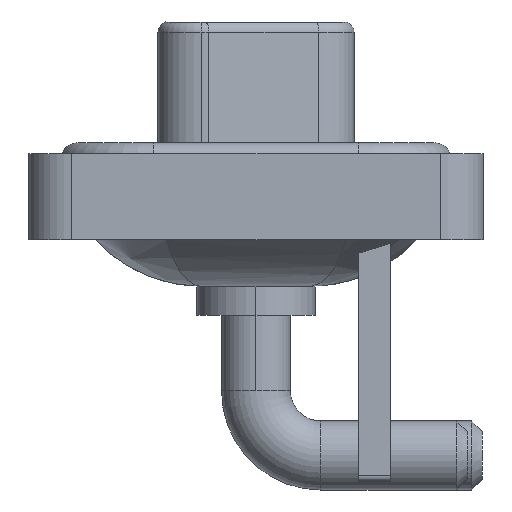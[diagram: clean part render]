
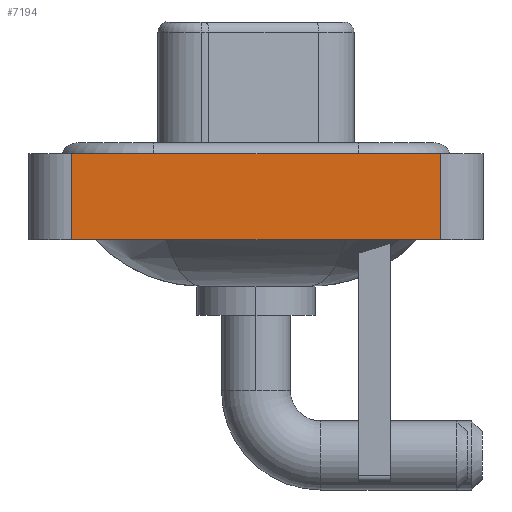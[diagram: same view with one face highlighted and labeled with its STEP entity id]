
A CAD part, left-side view. The second image highlights one B-rep face of the part: STEP entity #7194.
In plain terms, the highlighted planar face has unit normal (-1, 0, 0).
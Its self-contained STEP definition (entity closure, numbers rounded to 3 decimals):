
#233 = CARTESIAN_POINT ( 'NONE',  ( -7.3, -8.55, 0.4 ) ) ;
#431 = CARTESIAN_POINT ( 'NONE',  ( -7.3, 8.55, -3.6 ) ) ;
#856 = DIRECTION ( 'NONE',  ( 0., 0., 1. ) ) ;
#1023 = VECTOR ( 'NONE', #856, 1000. ) ;
#2092 = AXIS2_PLACEMENT_3D ( 'NONE', #8544, #11675, #17555 ) ;
#2222 = CARTESIAN_POINT ( 'NONE',  ( -7.3, -8.55, -3.6 ) ) ;
#2843 = EDGE_LOOP ( 'NONE', ( #18451, #3415, #3178, #11328 ) ) ;
#2860 = CARTESIAN_POINT ( 'NONE',  ( -7.3, 8.55, -3.6 ) ) ;
#2869 = CARTESIAN_POINT ( 'NONE',  ( -7.3, -8.55, -3.6 ) ) ;
#3178 = ORIENTED_EDGE ( 'NONE', *, *, #15656, .F. ) ;
#3415 = ORIENTED_EDGE ( 'NONE', *, *, #11580, .F. ) ;
#3864 = DIRECTION ( 'NONE',  ( 0., 0., 1. ) ) ;
#5743 = VECTOR ( 'NONE', #16312, 1000. ) ;
#6974 = VERTEX_POINT ( 'NONE', #2869 ) ;
#7194 = ADVANCED_FACE ( 'NONE', ( #16338 ), #14926, .T. ) ;
#8317 = VERTEX_POINT ( 'NONE', #431 ) ;
#8418 = VERTEX_POINT ( 'NONE', #9758 ) ;
#8544 = CARTESIAN_POINT ( 'NONE',  ( -7.3, -8.55, -3.6 ) ) ;
#9758 = CARTESIAN_POINT ( 'NONE',  ( -7.3, -8.55, 0.4 ) ) ;
#10159 = VECTOR ( 'NONE', #14210, 1000. ) ;
#10348 = EDGE_CURVE ( 'NONE', #8317, #6974, #19067, .T. ) ;
#11328 = ORIENTED_EDGE ( 'NONE', *, *, #10348, .T. ) ;
#11378 = CARTESIAN_POINT ( 'NONE',  ( -7.3, 8.55, 0.4 ) ) ;
#11580 = EDGE_CURVE ( 'NONE', #19801, #8418, #15632, .T. ) ;
#11675 = DIRECTION ( 'NONE',  ( -1., 0., 0. ) ) ;
#12478 = CARTESIAN_POINT ( 'NONE',  ( -7.3, -8.55, -3.6 ) ) ;
#14210 = DIRECTION ( 'NONE',  ( 0., -1., 0. ) ) ;
#14926 = PLANE ( 'NONE',  #2092 ) ;
#14942 = EDGE_CURVE ( 'NONE', #6974, #8418, #17750, .T. ) ;
#15632 = LINE ( 'NONE', #233, #10159 ) ;
#15656 = EDGE_CURVE ( 'NONE', #8317, #19801, #16745, .T. ) ;
#16312 = DIRECTION ( 'NONE',  ( 0., -1., 0. ) ) ;
#16338 = FACE_OUTER_BOUND ( 'NONE', #2843, .T. ) ;
#16745 = LINE ( 'NONE', #2860, #1023 ) ;
#16843 = VECTOR ( 'NONE', #3864, 1000. ) ;
#17555 = DIRECTION ( 'NONE',  ( 0., 0., 1. ) ) ;
#17750 = LINE ( 'NONE', #2222, #16843 ) ;
#18451 = ORIENTED_EDGE ( 'NONE', *, *, #14942, .T. ) ;
#19067 = LINE ( 'NONE', #12478, #5743 ) ;
#19801 = VERTEX_POINT ( 'NONE', #11378 ) ;
